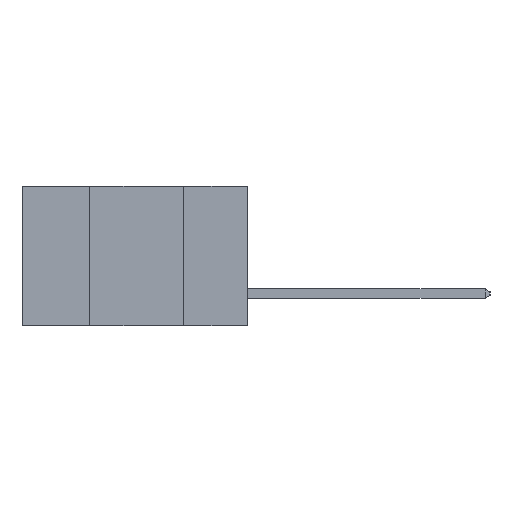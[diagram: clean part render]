
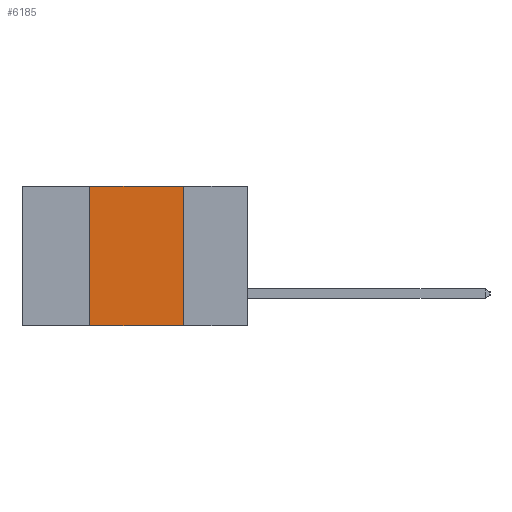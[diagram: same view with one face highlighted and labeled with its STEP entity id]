
A CAD part, left-side view. The second image highlights one B-rep face of the part: STEP entity #6185.
In plain terms, the highlighted planar face has unit normal (-1, 0, 0).
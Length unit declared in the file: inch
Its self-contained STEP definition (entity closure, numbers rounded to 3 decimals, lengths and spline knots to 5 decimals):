
#409 = LINE ( 'NONE', #15297, #15796 ) ;
#689 = ORIENTED_EDGE ( 'NONE', *, *, #24572, .F. ) ;
#2339 = VERTEX_POINT ( 'NONE', #20066 ) ;
#2613 = VERTEX_POINT ( 'NONE', #24328 ) ;
#3204 = ORIENTED_EDGE ( 'NONE', *, *, #6338, .F. ) ;
#3784 = VERTEX_POINT ( 'NONE', #10956 ) ;
#3849 = ORIENTED_EDGE ( 'NONE', *, *, #12180, .F. ) ;
#3982 = EDGE_LOOP ( 'NONE', ( #3849, #3204, #689, #14446 ) ) ;
#6102 = DIRECTION ( 'NONE',  ( 0., 0., 1. ) ) ;
#6185 = ADVANCED_FACE ( 'NONE', ( #8836 ), #17784, .F. ) ;
#6338 = EDGE_CURVE ( 'NONE', #2613, #2339, #409, .T. ) ;
#7371 = CARTESIAN_POINT ( 'NONE',  ( 0., 0.6, -0.37 ) ) ;
#7533 = CARTESIAN_POINT ( 'NONE',  ( 0., 0.17, -0.37 ) ) ;
#8836 = FACE_OUTER_BOUND ( 'NONE', #3982, .T. ) ;
#9260 = VECTOR ( 'NONE', #21409, 39.37008 ) ;
#10956 = CARTESIAN_POINT ( 'NONE',  ( 0., 0.42, -0.37 ) ) ;
#11613 = AXIS2_PLACEMENT_3D ( 'NONE', #17613, #17575, #17495 ) ;
#12180 = EDGE_CURVE ( 'NONE', #2339, #14060, #14436, .T. ) ;
#14060 = VERTEX_POINT ( 'NONE', #7533 ) ;
#14436 = LINE ( 'NONE', #15705, #24412 ) ;
#14446 = ORIENTED_EDGE ( 'NONE', *, *, #22765, .T. ) ;
#15259 = DIRECTION ( 'NONE',  ( 0., -1., 0. ) ) ;
#15297 = CARTESIAN_POINT ( 'NONE',  ( 0., 0.6, 0. ) ) ;
#15705 = CARTESIAN_POINT ( 'NONE',  ( 0., 0.17, -0.37 ) ) ;
#15796 = VECTOR ( 'NONE', #15259, 39.37008 ) ;
#15799 = VECTOR ( 'NONE', #6102, 39.37008 ) ;
#16129 = CARTESIAN_POINT ( 'NONE',  ( 0., 0.42, -0.37 ) ) ;
#17495 = DIRECTION ( 'NONE',  ( 0., 0., -1. ) ) ;
#17575 = DIRECTION ( 'NONE',  ( 1., 0., 0. ) ) ;
#17613 = CARTESIAN_POINT ( 'NONE',  ( 0., 0.6, 0. ) ) ;
#17746 = DIRECTION ( 'NONE',  ( 0., 0., -1. ) ) ;
#17784 = PLANE ( 'NONE',  #11613 ) ;
#18739 = LINE ( 'NONE', #7371, #9260 ) ;
#20066 = CARTESIAN_POINT ( 'NONE',  ( 0., 0.17, 0. ) ) ;
#21106 = LINE ( 'NONE', #16129, #15799 ) ;
#21409 = DIRECTION ( 'NONE',  ( 0., -1., 0. ) ) ;
#22765 = EDGE_CURVE ( 'NONE', #3784, #14060, #18739, .T. ) ;
#24328 = CARTESIAN_POINT ( 'NONE',  ( 0., 0.42, 0. ) ) ;
#24412 = VECTOR ( 'NONE', #17746, 39.37008 ) ;
#24572 = EDGE_CURVE ( 'NONE', #3784, #2613, #21106, .T. ) ;
